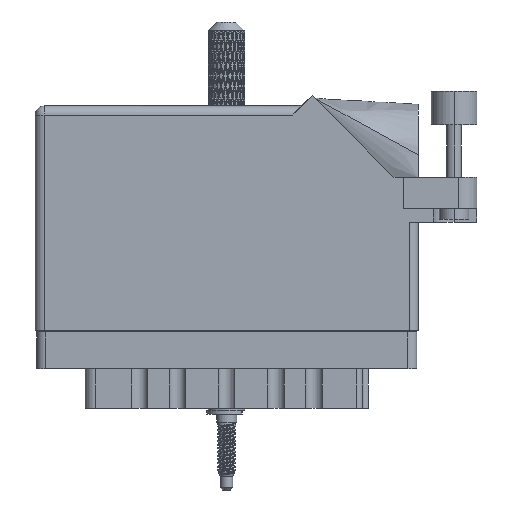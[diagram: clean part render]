
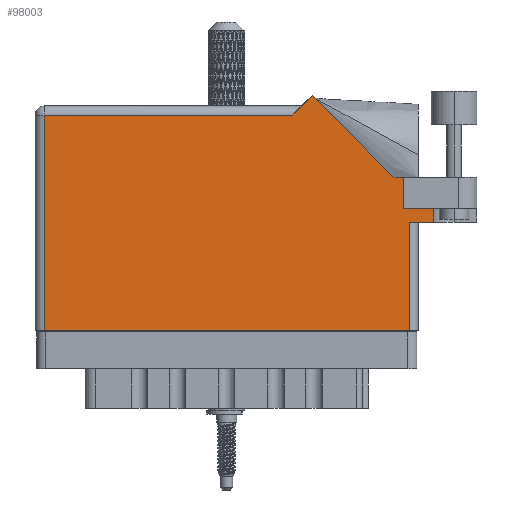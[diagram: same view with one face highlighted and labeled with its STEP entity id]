
A CAD part, front view. The second image highlights one B-rep face of the part: STEP entity #98003.
In plain terms, the highlighted face is planar.
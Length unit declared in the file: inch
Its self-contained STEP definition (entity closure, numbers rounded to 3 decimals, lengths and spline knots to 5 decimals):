
#240 = EDGE_CURVE ( 'NONE', #56739, #62365, #18698, .T. ) ;
#760 = VECTOR ( 'NONE', #107028, 39.37008 ) ;
#6122 = CARTESIAN_POINT ( 'NONE',  ( 2.7135, 0.737, 0. ) ) ;
#6149 = CARTESIAN_POINT ( 'NONE',  ( 2.512, 1.044, 0. ) ) ;
#7492 = EDGE_CURVE ( 'NONE', #109364, #99254, #109357, .T. ) ;
#7738 = LINE ( 'NONE', #9021, #107837 ) ;
#7926 = DIRECTION ( 'NONE',  ( 0., 0., -1. ) ) ;
#8694 = ORIENTED_EDGE ( 'NONE', *, *, #115295, .T. ) ;
#9021 = CARTESIAN_POINT ( 'NONE',  ( 2.44642, 1.044, 0. ) ) ;
#11084 = EDGE_CURVE ( 'NONE', #99254, #102925, #79735, .T. ) ;
#11363 = ORIENTED_EDGE ( 'NONE', *, *, #7492, .T. ) ;
#11547 = CARTESIAN_POINT ( 'NONE',  ( 2.7135, 0.831, 0. ) ) ;
#11791 = VECTOR ( 'NONE', #48450, 39.37008 ) ;
#13158 = CARTESIAN_POINT ( 'NONE',  ( 2.55, 0.737, 0. ) ) ;
#16851 = EDGE_CURVE ( 'NONE', #102925, #72309, #75066, .T. ) ;
#18081 = VERTEX_POINT ( 'NONE', #75634 ) ;
#18698 = LINE ( 'NONE', #34794, #89575 ) ;
#21804 = CARTESIAN_POINT ( 'NONE',  ( 2.55, 0., 0. ) ) ;
#22998 = VERTEX_POINT ( 'NONE', #13158 ) ;
#23219 = EDGE_CURVE ( 'NONE', #87760, #79251, #40630, .T. ) ;
#25196 = CARTESIAN_POINT ( 'NONE',  ( 2.512, 0.831, 0. ) ) ;
#26248 = VECTOR ( 'NONE', #69171, 39.37008 ) ;
#26748 = CARTESIAN_POINT ( 'NONE',  ( 0., 1.468, 0. ) ) ;
#32961 = VECTOR ( 'NONE', #70626, 39.37008 ) ;
#34794 = CARTESIAN_POINT ( 'NONE',  ( 2.7135, 1.16177, 0. ) ) ;
#35526 = DIRECTION ( 'NONE',  ( -0.707, 0.707, 0. ) ) ;
#37575 = ORIENTED_EDGE ( 'NONE', *, *, #53166, .F. ) ;
#38361 = VECTOR ( 'NONE', #47836, 39.37008 ) ;
#40630 = LINE ( 'NONE', #25196, #111505 ) ;
#47836 = DIRECTION ( 'NONE',  ( 0., 1., 0. ) ) ;
#48450 = DIRECTION ( 'NONE',  ( -1., 0., 0. ) ) ;
#49034 = CARTESIAN_POINT ( 'NONE',  ( 2.512, 0.831, 0. ) ) ;
#51490 = ORIENTED_EDGE ( 'NONE', *, *, #68459, .T. ) ;
#52614 = LINE ( 'NONE', #114241, #26248 ) ;
#53166 = EDGE_CURVE ( 'NONE', #87760, #56739, #112108, .T. ) ;
#53345 = DIRECTION ( 'NONE',  ( 0., -1., 0. ) ) ;
#53411 = CARTESIAN_POINT ( 'NONE',  ( 0.062, 1.468, 0. ) ) ;
#54802 = DIRECTION ( 'NONE',  ( 0., -1., 0. ) ) ;
#56737 = DIRECTION ( 'NONE',  ( -0.707, -0.707, 0. ) ) ;
#56739 = VERTEX_POINT ( 'NONE', #11547 ) ;
#60499 = VECTOR ( 'NONE', #56737, 39.37008 ) ;
#60793 = CARTESIAN_POINT ( 'NONE',  ( 0., 1.53, 0. ) ) ;
#61917 = LINE ( 'NONE', #82075, #60499 ) ;
#62365 = VERTEX_POINT ( 'NONE', #6122 ) ;
#65915 = CARTESIAN_POINT ( 'NONE',  ( 0., 0., 0. ) ) ;
#66037 = CARTESIAN_POINT ( 'NONE',  ( 2.55, 0.737, 0. ) ) ;
#66245 = CARTESIAN_POINT ( 'NONE',  ( 1.757, 1.468, 0. ) ) ;
#68459 = EDGE_CURVE ( 'NONE', #89424, #18081, #7738, .T. ) ;
#69171 = DIRECTION ( 'NONE',  ( 1., 0., 0. ) ) ;
#70184 = ORIENTED_EDGE ( 'NONE', *, *, #114960, .T. ) ;
#70626 = DIRECTION ( 'NONE',  ( -1., 0., 0. ) ) ;
#72236 = VECTOR ( 'NONE', #92765, 39.37008 ) ;
#72309 = VERTEX_POINT ( 'NONE', #21804 ) ;
#74477 = LINE ( 'NONE', #66037, #38361 ) ;
#75066 = LINE ( 'NONE', #65915, #72236 ) ;
#75634 = CARTESIAN_POINT ( 'NONE',  ( 1.88971, 1.60071, 0. ) ) ;
#76360 = EDGE_CURVE ( 'NONE', #22998, #62365, #52614, .T. ) ;
#76414 = FACE_OUTER_BOUND ( 'NONE', #100042, .T. ) ;
#77150 = LINE ( 'NONE', #84639, #11791 ) ;
#79251 = VERTEX_POINT ( 'NONE', #6149 ) ;
#79735 = LINE ( 'NONE', #108033, #106144 ) ;
#82075 = CARTESIAN_POINT ( 'NONE',  ( 1.819, 1.53, 0. ) ) ;
#84639 = CARTESIAN_POINT ( 'NONE',  ( 3.012, 1.044, 0. ) ) ;
#86924 = CARTESIAN_POINT ( 'NONE',  ( 0.062, 0., 0. ) ) ;
#87317 = DIRECTION ( 'NONE',  ( 0., 1., 0. ) ) ;
#87760 = VERTEX_POINT ( 'NONE', #49034 ) ;
#89424 = VERTEX_POINT ( 'NONE', #92811 ) ;
#89575 = VECTOR ( 'NONE', #53345, 39.37008 ) ;
#90486 = ORIENTED_EDGE ( 'NONE', *, *, #114894, .T. ) ;
#91175 = ORIENTED_EDGE ( 'NONE', *, *, #16851, .T. ) ;
#92202 = ORIENTED_EDGE ( 'NONE', *, *, #76360, .T. ) ;
#92765 = DIRECTION ( 'NONE',  ( 1., 0., 0. ) ) ;
#92811 = CARTESIAN_POINT ( 'NONE',  ( 2.44642, 1.044, 0. ) ) ;
#93145 = ORIENTED_EDGE ( 'NONE', *, *, #23219, .T. ) ;
#93984 = AXIS2_PLACEMENT_3D ( 'NONE', #60793, #7926, #103971 ) ;
#96197 = PLANE ( 'NONE',  #93984 ) ;
#98003 = ADVANCED_FACE ( 'NONE', ( #76414 ), #96197, .F. ) ;
#98045 = CARTESIAN_POINT ( 'NONE',  ( 2.512, 0.831, 0. ) ) ;
#98111 = ORIENTED_EDGE ( 'NONE', *, *, #11084, .T. ) ;
#99254 = VERTEX_POINT ( 'NONE', #53411 ) ;
#100042 = EDGE_LOOP ( 'NONE', ( #91175, #70184, #92202, #104156, #37575, #93145, #8694, #51490, #90486, #11363, #98111 ) ) ;
#102925 = VERTEX_POINT ( 'NONE', #86924 ) ;
#103971 = DIRECTION ( 'NONE',  ( -1., 0., 0. ) ) ;
#104156 = ORIENTED_EDGE ( 'NONE', *, *, #240, .F. ) ;
#106144 = VECTOR ( 'NONE', #54802, 39.37008 ) ;
#107028 = DIRECTION ( 'NONE',  ( 1., 0., 0. ) ) ;
#107837 = VECTOR ( 'NONE', #35526, 39.37008 ) ;
#108033 = CARTESIAN_POINT ( 'NONE',  ( 0.062, 0., 0. ) ) ;
#109357 = LINE ( 'NONE', #26748, #32961 ) ;
#109364 = VERTEX_POINT ( 'NONE', #66245 ) ;
#111505 = VECTOR ( 'NONE', #87317, 39.37008 ) ;
#112108 = LINE ( 'NONE', #98045, #760 ) ;
#114241 = CARTESIAN_POINT ( 'NONE',  ( 2.612, 0.737, 0. ) ) ;
#114894 = EDGE_CURVE ( 'NONE', #18081, #109364, #61917, .T. ) ;
#114960 = EDGE_CURVE ( 'NONE', #72309, #22998, #74477, .T. ) ;
#115295 = EDGE_CURVE ( 'NONE', #79251, #89424, #77150, .T. ) ;
